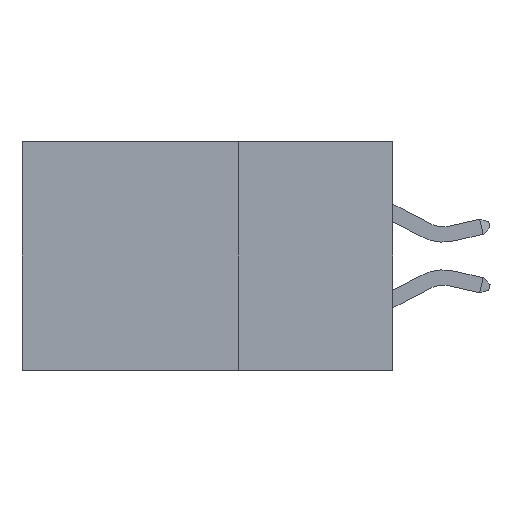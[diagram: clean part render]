
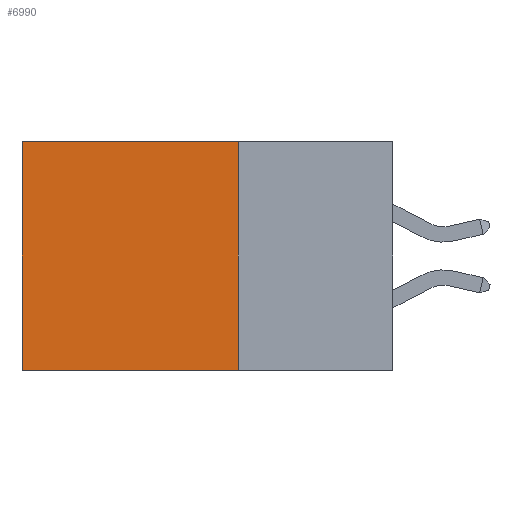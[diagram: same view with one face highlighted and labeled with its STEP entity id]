
A CAD part, left-side view. The second image highlights one B-rep face of the part: STEP entity #6990.
In plain terms, the highlighted planar face has unit normal (-1, 0, 0).
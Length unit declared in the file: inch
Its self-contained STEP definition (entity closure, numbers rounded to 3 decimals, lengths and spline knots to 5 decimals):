
#865 = CARTESIAN_POINT ( 'NONE',  ( 0.2875, 0.25, 0. ) ) ;
#1532 = ORIENTED_EDGE ( 'NONE', *, *, #5075, .T. ) ;
#1860 = CARTESIAN_POINT ( 'NONE',  ( 0.2875, 0.25, -0.37 ) ) ;
#2279 = LINE ( 'NONE', #24024, #4337 ) ;
#4056 = DIRECTION ( 'NONE',  ( 1., 0., 0. ) ) ;
#4188 = DIRECTION ( 'NONE',  ( 0., 1., 0. ) ) ;
#4305 = VECTOR ( 'NONE', #14364, 39.37008 ) ;
#4337 = VECTOR ( 'NONE', #4502, 39.37008 ) ;
#4502 = DIRECTION ( 'NONE',  ( 0., 0., -1. ) ) ;
#4679 = VERTEX_POINT ( 'NONE', #12507 ) ;
#5075 = EDGE_CURVE ( 'NONE', #4679, #36685, #21674, .T. ) ;
#6990 = ADVANCED_FACE ( 'NONE', ( #40241 ), #13789, .F. ) ;
#7654 = ORIENTED_EDGE ( 'NONE', *, *, #28790, .F. ) ;
#9377 = EDGE_CURVE ( 'NONE', #15999, #28456, #2279, .T. ) ;
#10082 = ORIENTED_EDGE ( 'NONE', *, *, #9377, .F. ) ;
#11038 = CARTESIAN_POINT ( 'NONE',  ( 0.2875, 0.6, 0. ) ) ;
#12507 = CARTESIAN_POINT ( 'NONE',  ( 0.2875, 0.6, 0. ) ) ;
#13024 = LINE ( 'NONE', #1860, #37953 ) ;
#13634 = VECTOR ( 'NONE', #4188, 39.37008 ) ;
#13789 = PLANE ( 'NONE',  #24937 ) ;
#14364 = DIRECTION ( 'NONE',  ( 0., 0., -1. ) ) ;
#15999 = VERTEX_POINT ( 'NONE', #31483 ) ;
#16793 = ORIENTED_EDGE ( 'NONE', *, *, #23977, .T. ) ;
#21438 = DIRECTION ( 'NONE',  ( 0., 1., 0. ) ) ;
#21674 = LINE ( 'NONE', #11038, #4305 ) ;
#23593 = CARTESIAN_POINT ( 'NONE',  ( 0.2875, 0.25, 0. ) ) ;
#23977 = EDGE_CURVE ( 'NONE', #15999, #4679, #37544, .T. ) ;
#24024 = CARTESIAN_POINT ( 'NONE',  ( 0.2875, 0.25, 0. ) ) ;
#24937 = AXIS2_PLACEMENT_3D ( 'NONE', #23593, #4056, #26865 ) ;
#26865 = DIRECTION ( 'NONE',  ( 0., 0., -1. ) ) ;
#28456 = VERTEX_POINT ( 'NONE', #39201 ) ;
#28790 = EDGE_CURVE ( 'NONE', #28456, #36685, #13024, .T. ) ;
#31483 = CARTESIAN_POINT ( 'NONE',  ( 0.2875, 0.25, 0. ) ) ;
#31832 = EDGE_LOOP ( 'NONE', ( #1532, #7654, #10082, #16793 ) ) ;
#36685 = VERTEX_POINT ( 'NONE', #40150 ) ;
#37544 = LINE ( 'NONE', #865, #13634 ) ;
#37953 = VECTOR ( 'NONE', #21438, 39.37008 ) ;
#39201 = CARTESIAN_POINT ( 'NONE',  ( 0.2875, 0.25, -0.37 ) ) ;
#40150 = CARTESIAN_POINT ( 'NONE',  ( 0.2875, 0.6, -0.37 ) ) ;
#40241 = FACE_OUTER_BOUND ( 'NONE', #31832, .T. ) ;
